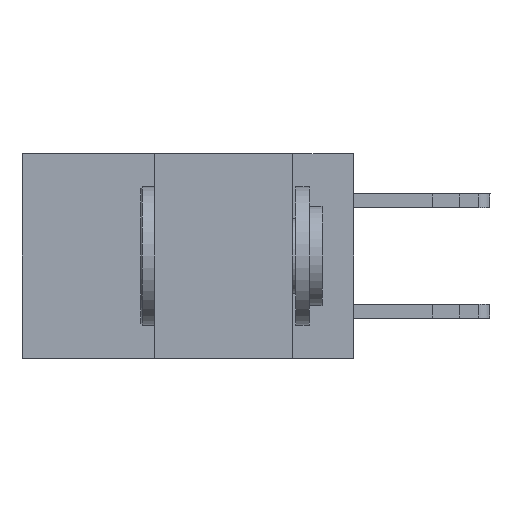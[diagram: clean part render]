
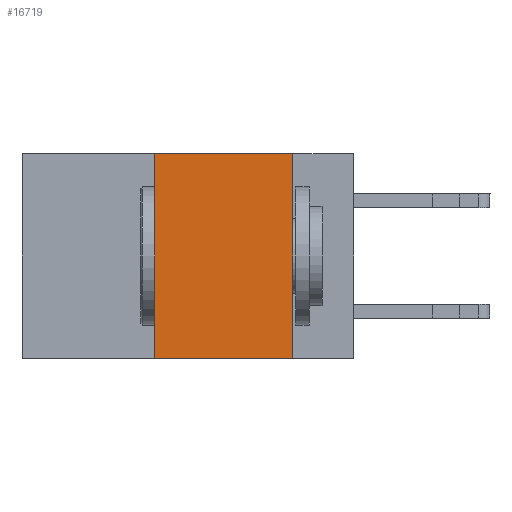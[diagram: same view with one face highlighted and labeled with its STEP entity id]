
A CAD part, left-side view. The second image highlights one B-rep face of the part: STEP entity #16719.
In plain terms, the highlighted planar face has unit normal (-1, 0, 0).
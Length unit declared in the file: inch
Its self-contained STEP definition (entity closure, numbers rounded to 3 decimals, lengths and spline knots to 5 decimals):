
#698 = AXIS2_PLACEMENT_3D ( 'NONE', #18738, #6099, #7752 ) ;
#754 = VECTOR ( 'NONE', #10265, 39.37008 ) ;
#1000 = ORIENTED_EDGE ( 'NONE', *, *, #13525, .T. ) ;
#2986 = EDGE_CURVE ( 'NONE', #9533, #11795, #10368, .T. ) ;
#3527 = CARTESIAN_POINT ( 'NONE',  ( 0., 0.11, -0.37 ) ) ;
#5888 = CARTESIAN_POINT ( 'NONE',  ( 0., 0.36, 0. ) ) ;
#5986 = CARTESIAN_POINT ( 'NONE',  ( 0., 0.11, 0. ) ) ;
#6099 = DIRECTION ( 'NONE',  ( 1., 0., 0. ) ) ;
#6675 = CARTESIAN_POINT ( 'NONE',  ( 0., 0.6, -0.37 ) ) ;
#7752 = DIRECTION ( 'NONE',  ( 0., 0., -1. ) ) ;
#7966 = DIRECTION ( 'NONE',  ( 0., 0., -1. ) ) ;
#8104 = CARTESIAN_POINT ( 'NONE',  ( 0., 0.6, 0. ) ) ;
#8812 = ORIENTED_EDGE ( 'NONE', *, *, #13877, .F. ) ;
#9533 = VERTEX_POINT ( 'NONE', #5986 ) ;
#9792 = ORIENTED_EDGE ( 'NONE', *, *, #15015, .F. ) ;
#10046 = LINE ( 'NONE', #6675, #14356 ) ;
#10265 = DIRECTION ( 'NONE',  ( 0., 0., 1. ) ) ;
#10368 = LINE ( 'NONE', #10778, #10839 ) ;
#10778 = CARTESIAN_POINT ( 'NONE',  ( 0., 0.11, 0. ) ) ;
#10839 = VECTOR ( 'NONE', #7966, 39.37008 ) ;
#11435 = CARTESIAN_POINT ( 'NONE',  ( 0., 0.36, 0. ) ) ;
#11593 = VECTOR ( 'NONE', #18201, 39.37008 ) ;
#11795 = VERTEX_POINT ( 'NONE', #3527 ) ;
#12869 = FACE_OUTER_BOUND ( 'NONE', #17090, .T. ) ;
#13525 = EDGE_CURVE ( 'NONE', #16228, #11795, #10046, .T. ) ;
#13801 = VERTEX_POINT ( 'NONE', #11435 ) ;
#13877 = EDGE_CURVE ( 'NONE', #16228, #13801, #16152, .T. ) ;
#14356 = VECTOR ( 'NONE', #17820, 39.37008 ) ;
#14386 = PLANE ( 'NONE',  #698 ) ;
#15015 = EDGE_CURVE ( 'NONE', #13801, #9533, #18369, .T. ) ;
#16152 = LINE ( 'NONE', #5888, #754 ) ;
#16228 = VERTEX_POINT ( 'NONE', #16609 ) ;
#16456 = ORIENTED_EDGE ( 'NONE', *, *, #2986, .F. ) ;
#16609 = CARTESIAN_POINT ( 'NONE',  ( 0., 0.36, -0.37 ) ) ;
#16719 = ADVANCED_FACE ( 'NONE', ( #12869 ), #14386, .F. ) ;
#17090 = EDGE_LOOP ( 'NONE', ( #16456, #9792, #8812, #1000 ) ) ;
#17820 = DIRECTION ( 'NONE',  ( 0., -1., 0. ) ) ;
#18201 = DIRECTION ( 'NONE',  ( 0., -1., 0. ) ) ;
#18369 = LINE ( 'NONE', #8104, #11593 ) ;
#18738 = CARTESIAN_POINT ( 'NONE',  ( 0., 0.6, 0. ) ) ;
